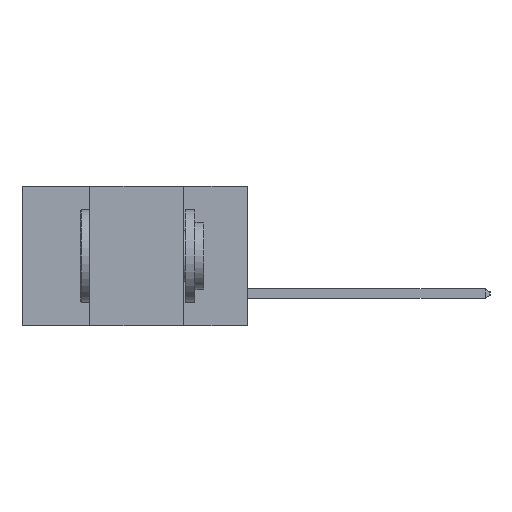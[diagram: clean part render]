
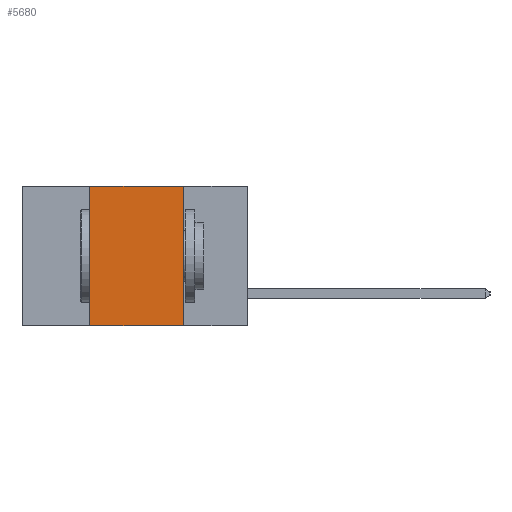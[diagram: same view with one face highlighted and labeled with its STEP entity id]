
A CAD part, left-side view. The second image highlights one B-rep face of the part: STEP entity #5680.
In plain terms, the highlighted planar face has unit normal (-1, 0, 0).
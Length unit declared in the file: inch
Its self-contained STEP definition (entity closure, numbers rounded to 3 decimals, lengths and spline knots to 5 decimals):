
#48 = ORIENTED_EDGE ( 'NONE', *, *, #6113, .F. ) ;
#367 = CARTESIAN_POINT ( 'NONE',  ( 0., 0.6, -0.37 ) ) ;
#809 = DIRECTION ( 'NONE',  ( 0., -1., 0. ) ) ;
#1138 = VERTEX_POINT ( 'NONE', #15702 ) ;
#1409 = CARTESIAN_POINT ( 'NONE',  ( 0., 0.6, 0. ) ) ;
#1950 = EDGE_CURVE ( 'NONE', #11205, #4292, #11545, .T. ) ;
#2342 = ORIENTED_EDGE ( 'NONE', *, *, #7475, .F. ) ;
#2526 = EDGE_CURVE ( 'NONE', #1138, #13516, #11769, .T. ) ;
#2830 = VECTOR ( 'NONE', #17737, 39.37008 ) ;
#2901 = DIRECTION ( 'NONE',  ( 0., -1., 0. ) ) ;
#3415 = ORIENTED_EDGE ( 'NONE', *, *, #2526, .F. ) ;
#3449 = LINE ( 'NONE', #4613, #15976 ) ;
#3476 = AXIS2_PLACEMENT_3D ( 'NONE', #9239, #9167, #9149 ) ;
#4292 = VERTEX_POINT ( 'NONE', #5939 ) ;
#4569 = DIRECTION ( 'NONE',  ( 0., 0., -1. ) ) ;
#4613 = CARTESIAN_POINT ( 'NONE',  ( 0., 0.17, -0.37 ) ) ;
#5172 = EDGE_LOOP ( 'NONE', ( #48, #3415, #2342, #14427 ) ) ;
#5680 = ADVANCED_FACE ( 'NONE', ( #20027 ), #9243, .F. ) ;
#5939 = CARTESIAN_POINT ( 'NONE',  ( 0., 0.17, -0.37 ) ) ;
#6113 = EDGE_CURVE ( 'NONE', #13516, #4292, #3449, .T. ) ;
#7475 = EDGE_CURVE ( 'NONE', #11205, #1138, #16449, .T. ) ;
#7481 = VECTOR ( 'NONE', #809, 39.37008 ) ;
#9149 = DIRECTION ( 'NONE',  ( 0., 0., -1. ) ) ;
#9167 = DIRECTION ( 'NONE',  ( 1., 0., 0. ) ) ;
#9239 = CARTESIAN_POINT ( 'NONE',  ( 0., 0.6, 0. ) ) ;
#9243 = PLANE ( 'NONE',  #3476 ) ;
#9604 = CARTESIAN_POINT ( 'NONE',  ( 0., 0.42, -0.37 ) ) ;
#10177 = CARTESIAN_POINT ( 'NONE',  ( 0., 0.17, 0. ) ) ;
#11205 = VERTEX_POINT ( 'NONE', #9604 ) ;
#11545 = LINE ( 'NONE', #367, #20168 ) ;
#11769 = LINE ( 'NONE', #1409, #7481 ) ;
#13516 = VERTEX_POINT ( 'NONE', #10177 ) ;
#14427 = ORIENTED_EDGE ( 'NONE', *, *, #1950, .T. ) ;
#15702 = CARTESIAN_POINT ( 'NONE',  ( 0., 0.42, 0. ) ) ;
#15976 = VECTOR ( 'NONE', #4569, 39.37008 ) ;
#16449 = LINE ( 'NONE', #17811, #2830 ) ;
#17737 = DIRECTION ( 'NONE',  ( 0., 0., 1. ) ) ;
#17811 = CARTESIAN_POINT ( 'NONE',  ( 0., 0.42, -0.37 ) ) ;
#20027 = FACE_OUTER_BOUND ( 'NONE', #5172, .T. ) ;
#20168 = VECTOR ( 'NONE', #2901, 39.37008 ) ;
